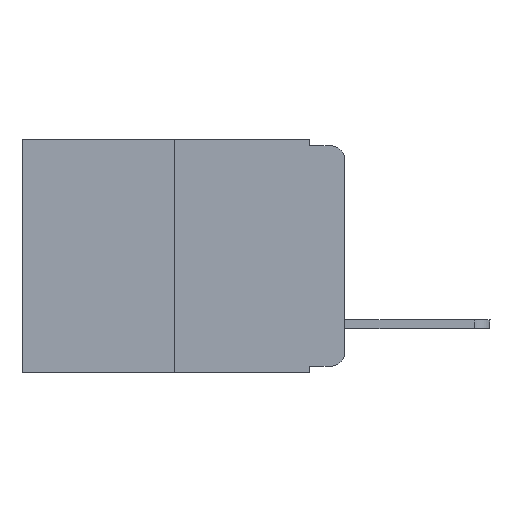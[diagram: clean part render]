
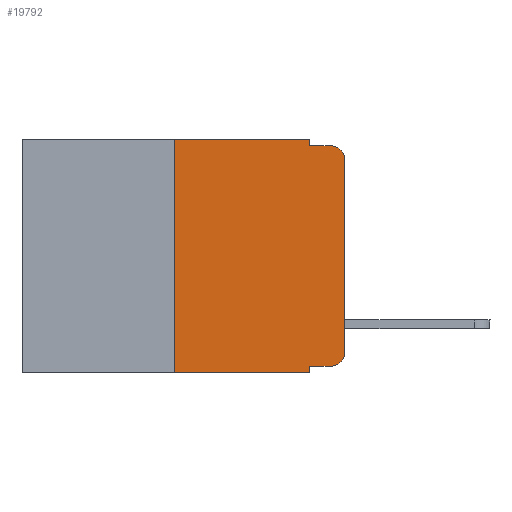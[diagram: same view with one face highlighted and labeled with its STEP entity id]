
A CAD part, left-side view. The second image highlights one B-rep face of the part: STEP entity #19792.
In plain terms, the highlighted planar face has unit normal (-1, 0, 0).
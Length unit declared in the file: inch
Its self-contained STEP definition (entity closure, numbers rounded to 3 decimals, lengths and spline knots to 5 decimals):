
#89 = DIRECTION ( 'NONE',  ( 0., 0., -1. ) ) ;
#241 = LINE ( 'NONE', #7641, #14761 ) ;
#314 = EDGE_CURVE ( 'NONE', #23525, #8140, #2366, .T. ) ;
#1230 = CARTESIAN_POINT ( 'NONE',  ( 0., 0.051, 0. ) ) ;
#1434 = ORIENTED_EDGE ( 'NONE', *, *, #1763, .T. ) ;
#1763 = EDGE_CURVE ( 'NONE', #16713, #2068, #8529, .T. ) ;
#2068 = VERTEX_POINT ( 'NONE', #10372 ) ;
#2240 = DIRECTION ( 'NONE',  ( 0., 0., -1. ) ) ;
#2366 = LINE ( 'NONE', #14783, #18312 ) ;
#3143 = CARTESIAN_POINT ( 'NONE',  ( 0., 0.051, 0. ) ) ;
#3158 = DIRECTION ( 'NONE',  ( 0., -1., 0. ) ) ;
#3965 = FACE_OUTER_BOUND ( 'NONE', #22620, .T. ) ;
#4219 = EDGE_CURVE ( 'NONE', #18760, #7250, #6558, .T. ) ;
#5061 = DIRECTION ( 'NONE',  ( -1., 0., 0. ) ) ;
#5078 = DIRECTION ( 'NONE',  ( 0., 0., -1. ) ) ;
#5246 = CARTESIAN_POINT ( 'NONE',  ( 0., 0.051, -0.343 ) ) ;
#5607 = EDGE_CURVE ( 'NONE', #8140, #5985, #241, .T. ) ;
#5644 = DIRECTION ( 'NONE',  ( 0., 0., 1. ) ) ;
#5985 = VERTEX_POINT ( 'NONE', #1230 ) ;
#6359 = VERTEX_POINT ( 'NONE', #22324 ) ;
#6558 = CIRCLE ( 'NONE', #12001, 0.02 ) ;
#7250 = VERTEX_POINT ( 'NONE', #15118 ) ;
#7279 = ORIENTED_EDGE ( 'NONE', *, *, #21066, .F. ) ;
#7365 = PLANE ( 'NONE',  #10872 ) ;
#7406 = DIRECTION ( 'NONE',  ( 0., -1., 0. ) ) ;
#7641 = CARTESIAN_POINT ( 'NONE',  ( 0., 0.473, 0. ) ) ;
#8140 = VERTEX_POINT ( 'NONE', #15511 ) ;
#8220 = ORIENTED_EDGE ( 'NONE', *, *, #4219, .T. ) ;
#8275 = CARTESIAN_POINT ( 'NONE',  ( 0., 0.25, -0.343 ) ) ;
#8483 = DIRECTION ( 'NONE',  ( 0., -1., 0. ) ) ;
#8529 = CIRCLE ( 'NONE', #11626, 0.02 ) ;
#9068 = DIRECTION ( 'NONE',  ( 0., 0., -1. ) ) ;
#9558 = CARTESIAN_POINT ( 'NONE',  ( 0., 0.051, 0. ) ) ;
#9643 = EDGE_CURVE ( 'NONE', #21758, #15758, #12642, .T. ) ;
#9695 = ORIENTED_EDGE ( 'NONE', *, *, #9643, .F. ) ;
#9708 = EDGE_CURVE ( 'NONE', #2068, #18760, #19661, .T. ) ;
#10372 = CARTESIAN_POINT ( 'NONE',  ( 0., 0., -0.313 ) ) ;
#10621 = CARTESIAN_POINT ( 'NONE',  ( 0., 0., -0.03 ) ) ;
#10758 = DIRECTION ( 'NONE',  ( -1., 0., 0. ) ) ;
#10872 = AXIS2_PLACEMENT_3D ( 'NONE', #14786, #16722, #89 ) ;
#11192 = DIRECTION ( 'NONE',  ( 0., -1., 0. ) ) ;
#11493 = ORIENTED_EDGE ( 'NONE', *, *, #314, .F. ) ;
#11626 = AXIS2_PLACEMENT_3D ( 'NONE', #18492, #10758, #9068 ) ;
#12001 = AXIS2_PLACEMENT_3D ( 'NONE', #14564, #5061, #12515 ) ;
#12336 = EDGE_CURVE ( 'NONE', #21758, #16713, #15527, .T. ) ;
#12515 = DIRECTION ( 'NONE',  ( 0., 0., -1. ) ) ;
#12642 = LINE ( 'NONE', #3143, #20202 ) ;
#12697 = VECTOR ( 'NONE', #8483, 39.37008 ) ;
#13251 = VECTOR ( 'NONE', #18200, 39.37008 ) ;
#14564 = CARTESIAN_POINT ( 'NONE',  ( 0., 0.02, -0.03 ) ) ;
#14761 = VECTOR ( 'NONE', #7406, 39.37008 ) ;
#14783 = CARTESIAN_POINT ( 'NONE',  ( 0., 0.25, 0. ) ) ;
#14786 = CARTESIAN_POINT ( 'NONE',  ( 0., 0.473, 0. ) ) ;
#14842 = LINE ( 'NONE', #22214, #21676 ) ;
#15118 = CARTESIAN_POINT ( 'NONE',  ( 0., 0.02, -0.01 ) ) ;
#15511 = CARTESIAN_POINT ( 'NONE',  ( 0., 0.25, 0. ) ) ;
#15527 = LINE ( 'NONE', #21349, #12697 ) ;
#15758 = VERTEX_POINT ( 'NONE', #5246 ) ;
#16122 = ORIENTED_EDGE ( 'NONE', *, *, #17635, .T. ) ;
#16420 = CARTESIAN_POINT ( 'NONE',  ( 0., 0.051, -0.01 ) ) ;
#16713 = VERTEX_POINT ( 'NONE', #22061 ) ;
#16722 = DIRECTION ( 'NONE',  ( 1., 0., 0. ) ) ;
#17260 = CARTESIAN_POINT ( 'NONE',  ( 0., 0.051, -0.333 ) ) ;
#17608 = ORIENTED_EDGE ( 'NONE', *, *, #12336, .T. ) ;
#17635 = EDGE_CURVE ( 'NONE', #23525, #15758, #14842, .T. ) ;
#18200 = DIRECTION ( 'NONE',  ( 0., 0., 1. ) ) ;
#18312 = VECTOR ( 'NONE', #5644, 39.37008 ) ;
#18492 = CARTESIAN_POINT ( 'NONE',  ( 0., 0.02, -0.313 ) ) ;
#18760 = VERTEX_POINT ( 'NONE', #10621 ) ;
#19423 = VECTOR ( 'NONE', #2240, 39.37008 ) ;
#19661 = LINE ( 'NONE', #20026, #13251 ) ;
#19721 = VECTOR ( 'NONE', #3158, 39.37008 ) ;
#19792 = ADVANCED_FACE ( 'NONE', ( #3965 ), #7365, .F. ) ;
#19800 = LINE ( 'NONE', #16420, #19721 ) ;
#20026 = CARTESIAN_POINT ( 'NONE',  ( 0., 0., 0. ) ) ;
#20202 = VECTOR ( 'NONE', #5078, 39.37008 ) ;
#20250 = LINE ( 'NONE', #9558, #19423 ) ;
#20453 = ORIENTED_EDGE ( 'NONE', *, *, #9708, .T. ) ;
#21066 = EDGE_CURVE ( 'NONE', #5985, #6359, #20250, .T. ) ;
#21349 = CARTESIAN_POINT ( 'NONE',  ( 0., 0.051, -0.333 ) ) ;
#21676 = VECTOR ( 'NONE', #11192, 39.37008 ) ;
#21758 = VERTEX_POINT ( 'NONE', #17260 ) ;
#21811 = ORIENTED_EDGE ( 'NONE', *, *, #23353, .F. ) ;
#22061 = CARTESIAN_POINT ( 'NONE',  ( 0., 0.02, -0.333 ) ) ;
#22214 = CARTESIAN_POINT ( 'NONE',  ( 0., 0.473, -0.343 ) ) ;
#22250 = ORIENTED_EDGE ( 'NONE', *, *, #5607, .F. ) ;
#22324 = CARTESIAN_POINT ( 'NONE',  ( 0., 0.051, -0.01 ) ) ;
#22620 = EDGE_LOOP ( 'NONE', ( #20453, #8220, #21811, #7279, #22250, #11493, #16122, #9695, #17608, #1434 ) ) ;
#23353 = EDGE_CURVE ( 'NONE', #6359, #7250, #19800, .T. ) ;
#23525 = VERTEX_POINT ( 'NONE', #8275 ) ;
